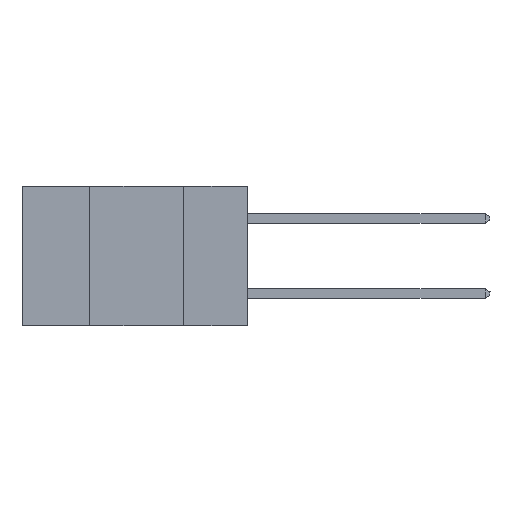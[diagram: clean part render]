
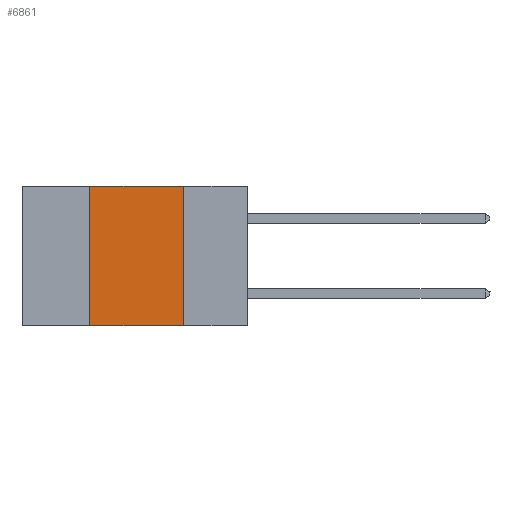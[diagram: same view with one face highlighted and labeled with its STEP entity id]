
A CAD part, left-side view. The second image highlights one B-rep face of the part: STEP entity #6861.
In plain terms, the highlighted planar face has unit normal (-1, 0, 0).
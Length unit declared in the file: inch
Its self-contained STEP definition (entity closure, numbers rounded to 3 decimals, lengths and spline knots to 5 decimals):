
#940 = ORIENTED_EDGE ( 'NONE', *, *, #6079, .F. ) ;
#1820 = CARTESIAN_POINT ( 'NONE',  ( 0., 0.6, 0. ) ) ;
#3272 = ORIENTED_EDGE ( 'NONE', *, *, #19625, .F. ) ;
#3682 = LINE ( 'NONE', #6298, #25751 ) ;
#3997 = DIRECTION ( 'NONE',  ( 1., 0., 0. ) ) ;
#5421 = VECTOR ( 'NONE', #19969, 39.37008 ) ;
#5429 = VERTEX_POINT ( 'NONE', #14129 ) ;
#6079 = EDGE_CURVE ( 'NONE', #24074, #5429, #16642, .T. ) ;
#6298 = CARTESIAN_POINT ( 'NONE',  ( 0., 0.42, -0.37 ) ) ;
#6861 = ADVANCED_FACE ( 'NONE', ( #24958 ), #16785, .F. ) ;
#7147 = CARTESIAN_POINT ( 'NONE',  ( 0., 0.42, -0.37 ) ) ;
#7238 = VERTEX_POINT ( 'NONE', #7147 ) ;
#8000 = DIRECTION ( 'NONE',  ( 0., 0., -1. ) ) ;
#8219 = LINE ( 'NONE', #12275, #18945 ) ;
#10032 = DIRECTION ( 'NONE',  ( 0., -1., 0. ) ) ;
#10846 = EDGE_CURVE ( 'NONE', #7238, #19637, #16788, .T. ) ;
#12275 = CARTESIAN_POINT ( 'NONE',  ( 0., 0.17, -0.37 ) ) ;
#14123 = EDGE_CURVE ( 'NONE', #5429, #19637, #8219, .T. ) ;
#14129 = CARTESIAN_POINT ( 'NONE',  ( 0., 0.17, 0. ) ) ;
#15674 = CARTESIAN_POINT ( 'NONE',  ( 0., 0.6, -0.37 ) ) ;
#16642 = LINE ( 'NONE', #27187, #21681 ) ;
#16785 = PLANE ( 'NONE',  #19402 ) ;
#16788 = LINE ( 'NONE', #15674, #5421 ) ;
#17039 = CARTESIAN_POINT ( 'NONE',  ( 0., 0.17, -0.37 ) ) ;
#17437 = ORIENTED_EDGE ( 'NONE', *, *, #10846, .T. ) ;
#18942 = DIRECTION ( 'NONE',  ( 0., 0., -1. ) ) ;
#18945 = VECTOR ( 'NONE', #8000, 39.37008 ) ;
#19402 = AXIS2_PLACEMENT_3D ( 'NONE', #1820, #3997, #18942 ) ;
#19625 = EDGE_CURVE ( 'NONE', #7238, #24074, #3682, .T. ) ;
#19637 = VERTEX_POINT ( 'NONE', #17039 ) ;
#19969 = DIRECTION ( 'NONE',  ( 0., -1., 0. ) ) ;
#21251 = DIRECTION ( 'NONE',  ( 0., 0., 1. ) ) ;
#21681 = VECTOR ( 'NONE', #10032, 39.37008 ) ;
#22518 = EDGE_LOOP ( 'NONE', ( #26907, #940, #3272, #17437 ) ) ;
#24074 = VERTEX_POINT ( 'NONE', #24830 ) ;
#24830 = CARTESIAN_POINT ( 'NONE',  ( 0., 0.42, 0. ) ) ;
#24958 = FACE_OUTER_BOUND ( 'NONE', #22518, .T. ) ;
#25751 = VECTOR ( 'NONE', #21251, 39.37008 ) ;
#26907 = ORIENTED_EDGE ( 'NONE', *, *, #14123, .F. ) ;
#27187 = CARTESIAN_POINT ( 'NONE',  ( 0., 0.6, 0. ) ) ;
